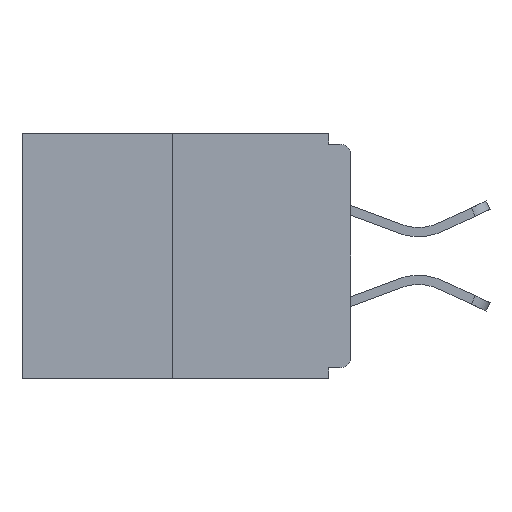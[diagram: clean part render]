
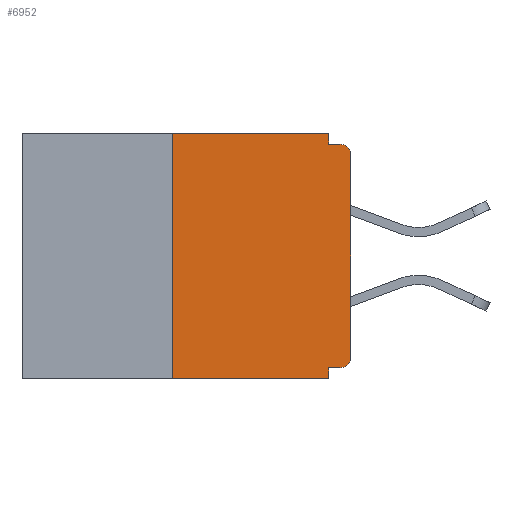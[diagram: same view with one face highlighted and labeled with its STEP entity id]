
A CAD part, left-side view. The second image highlights one B-rep face of the part: STEP entity #6952.
In plain terms, the highlighted planar face has unit normal (-1, 0, 0).
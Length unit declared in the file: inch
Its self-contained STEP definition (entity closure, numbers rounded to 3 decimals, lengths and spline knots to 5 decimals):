
#215 = CARTESIAN_POINT ( 'NONE',  ( 0., 0.031, -0.343 ) ) ;
#440 = DIRECTION ( 'NONE',  ( 0., 0., 1. ) ) ;
#488 = AXIS2_PLACEMENT_3D ( 'NONE', #24878, #8537, #24699 ) ;
#601 = ORIENTED_EDGE ( 'NONE', *, *, #12582, .F. ) ;
#1188 = EDGE_CURVE ( 'NONE', #5094, #3270, #25888, .T. ) ;
#3022 = FACE_OUTER_BOUND ( 'NONE', #9680, .T. ) ;
#3026 = CARTESIAN_POINT ( 'NONE',  ( 0., 0.031, 0. ) ) ;
#3068 = LINE ( 'NONE', #18588, #10121 ) ;
#3270 = VERTEX_POINT ( 'NONE', #14355 ) ;
#4931 = EDGE_CURVE ( 'NONE', #10763, #6494, #13921, .T. ) ;
#4947 = ORIENTED_EDGE ( 'NONE', *, *, #25625, .T. ) ;
#4981 = CARTESIAN_POINT ( 'NONE',  ( 0., 0.46, -0.343 ) ) ;
#5094 = VERTEX_POINT ( 'NONE', #13904 ) ;
#5548 = EDGE_CURVE ( 'NONE', #18585, #17074, #3068, .T. ) ;
#5600 = CIRCLE ( 'NONE', #7968, 0.015 ) ;
#5941 = CARTESIAN_POINT ( 'NONE',  ( 0., 0.031, -0.328 ) ) ;
#6494 = VERTEX_POINT ( 'NONE', #215 ) ;
#6952 = ADVANCED_FACE ( 'NONE', ( #3022 ), #18595, .F. ) ;
#7056 = ORIENTED_EDGE ( 'NONE', *, *, #1188, .T. ) ;
#7405 = ORIENTED_EDGE ( 'NONE', *, *, #5548, .F. ) ;
#7605 = VERTEX_POINT ( 'NONE', #21064 ) ;
#7968 = AXIS2_PLACEMENT_3D ( 'NONE', #11305, #15399, #17274 ) ;
#8045 = VECTOR ( 'NONE', #9337, 39.37008 ) ;
#8404 = CARTESIAN_POINT ( 'NONE',  ( 0., 0.25, 0. ) ) ;
#8537 = DIRECTION ( 'NONE',  ( 1., 0., 0. ) ) ;
#8996 = EDGE_CURVE ( 'NONE', #3270, #7605, #23642, .T. ) ;
#9323 = VERTEX_POINT ( 'NONE', #3026 ) ;
#9337 = DIRECTION ( 'NONE',  ( 0., -1., 0. ) ) ;
#9388 = DIRECTION ( 'NONE',  ( 0., 0., -1. ) ) ;
#9540 = LINE ( 'NONE', #25909, #10188 ) ;
#9680 = EDGE_LOOP ( 'NONE', ( #12758, #7405, #16328, #11957, #22217, #4947, #7056, #24306, #601, #14449 ) ) ;
#10104 = DIRECTION ( 'NONE',  ( -1., 0., 0. ) ) ;
#10113 = EDGE_CURVE ( 'NONE', #17074, #9323, #9540, .T. ) ;
#10121 = VECTOR ( 'NONE', #22711, 39.37008 ) ;
#10188 = VECTOR ( 'NONE', #21484, 39.37008 ) ;
#10221 = VECTOR ( 'NONE', #12249, 39.37008 ) ;
#10595 = VERTEX_POINT ( 'NONE', #13460 ) ;
#10763 = VERTEX_POINT ( 'NONE', #5941 ) ;
#10970 = CARTESIAN_POINT ( 'NONE',  ( 0., 0., 0. ) ) ;
#11305 = CARTESIAN_POINT ( 'NONE',  ( 0., 0.015, -0.313 ) ) ;
#11957 = ORIENTED_EDGE ( 'NONE', *, *, #4931, .F. ) ;
#12012 = VECTOR ( 'NONE', #21878, 39.37008 ) ;
#12249 = DIRECTION ( 'NONE',  ( 0., 1., 0. ) ) ;
#12582 = EDGE_CURVE ( 'NONE', #10595, #7605, #22213, .T. ) ;
#12758 = ORIENTED_EDGE ( 'NONE', *, *, #10113, .F. ) ;
#13460 = CARTESIAN_POINT ( 'NONE',  ( 0., 0.031, -0.015 ) ) ;
#13904 = CARTESIAN_POINT ( 'NONE',  ( 0., 0., -0.313 ) ) ;
#13921 = LINE ( 'NONE', #23286, #12012 ) ;
#14204 = CARTESIAN_POINT ( 'NONE',  ( 0., 0., -0.328 ) ) ;
#14355 = CARTESIAN_POINT ( 'NONE',  ( 0., 0., -0.03 ) ) ;
#14449 = ORIENTED_EDGE ( 'NONE', *, *, #19461, .F. ) ;
#15066 = EDGE_CURVE ( 'NONE', #18585, #6494, #24335, .T. ) ;
#15399 = DIRECTION ( 'NONE',  ( -1., 0., 0. ) ) ;
#15912 = CARTESIAN_POINT ( 'NONE',  ( 0., 0.015, -0.328 ) ) ;
#16328 = ORIENTED_EDGE ( 'NONE', *, *, #15066, .T. ) ;
#17074 = VERTEX_POINT ( 'NONE', #8404 ) ;
#17274 = DIRECTION ( 'NONE',  ( 0., 0., -1. ) ) ;
#18182 = VECTOR ( 'NONE', #440, 39.37008 ) ;
#18585 = VERTEX_POINT ( 'NONE', #24682 ) ;
#18588 = CARTESIAN_POINT ( 'NONE',  ( 0., 0.25, 0. ) ) ;
#18595 = PLANE ( 'NONE',  #488 ) ;
#18664 = VECTOR ( 'NONE', #19592, 39.37008 ) ;
#19461 = EDGE_CURVE ( 'NONE', #9323, #10595, #20570, .T. ) ;
#19504 = CARTESIAN_POINT ( 'NONE',  ( 0., 0., -0.015 ) ) ;
#19592 = DIRECTION ( 'NONE',  ( 0., -1., 0. ) ) ;
#20255 = VECTOR ( 'NONE', #9388, 39.37008 ) ;
#20570 = LINE ( 'NONE', #23946, #20255 ) ;
#21064 = CARTESIAN_POINT ( 'NONE',  ( 0., 0.015, -0.015 ) ) ;
#21484 = DIRECTION ( 'NONE',  ( 0., -1., 0. ) ) ;
#21878 = DIRECTION ( 'NONE',  ( 0., 0., -1. ) ) ;
#22213 = LINE ( 'NONE', #19504, #18664 ) ;
#22217 = ORIENTED_EDGE ( 'NONE', *, *, #23142, .F. ) ;
#22548 = AXIS2_PLACEMENT_3D ( 'NONE', #26202, #10104, #24475 ) ;
#22711 = DIRECTION ( 'NONE',  ( 0., 0., 1. ) ) ;
#22988 = VERTEX_POINT ( 'NONE', #15912 ) ;
#23142 = EDGE_CURVE ( 'NONE', #22988, #10763, #25890, .T. ) ;
#23286 = CARTESIAN_POINT ( 'NONE',  ( 0., 0.031, -0.343 ) ) ;
#23642 = CIRCLE ( 'NONE', #22548, 0.015 ) ;
#23946 = CARTESIAN_POINT ( 'NONE',  ( 0., 0.031, 0. ) ) ;
#24306 = ORIENTED_EDGE ( 'NONE', *, *, #8996, .T. ) ;
#24335 = LINE ( 'NONE', #4981, #8045 ) ;
#24475 = DIRECTION ( 'NONE',  ( 0., 0., -1. ) ) ;
#24682 = CARTESIAN_POINT ( 'NONE',  ( 0., 0.25, -0.343 ) ) ;
#24699 = DIRECTION ( 'NONE',  ( 0., 0., -1. ) ) ;
#24878 = CARTESIAN_POINT ( 'NONE',  ( 0., 0.46, 0. ) ) ;
#25625 = EDGE_CURVE ( 'NONE', #22988, #5094, #5600, .T. ) ;
#25888 = LINE ( 'NONE', #10970, #18182 ) ;
#25890 = LINE ( 'NONE', #14204, #10221 ) ;
#25909 = CARTESIAN_POINT ( 'NONE',  ( 0., 0.46, 0. ) ) ;
#26202 = CARTESIAN_POINT ( 'NONE',  ( 0., 0.015, -0.03 ) ) ;
